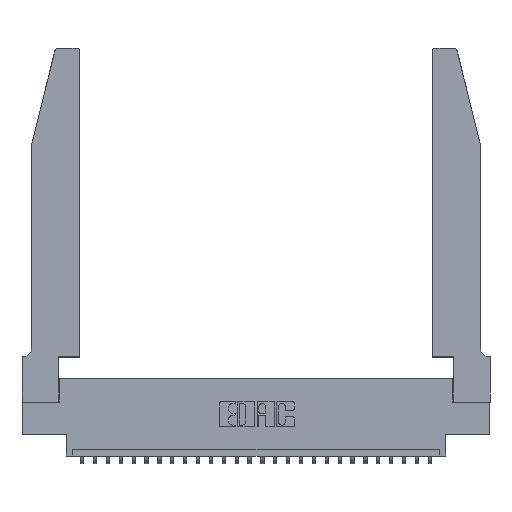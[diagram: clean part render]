
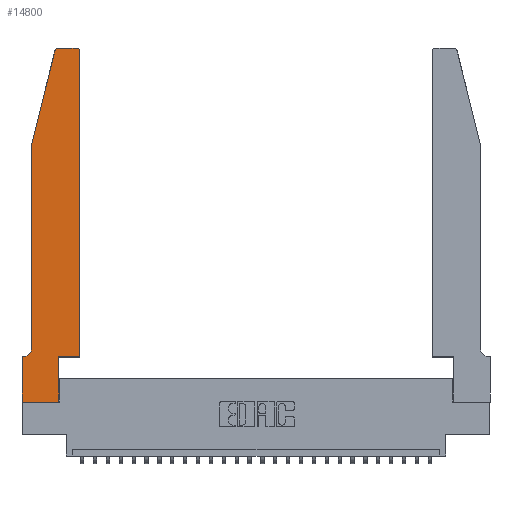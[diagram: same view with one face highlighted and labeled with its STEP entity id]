
A CAD part, top view. The second image highlights one B-rep face of the part: STEP entity #14800.
In plain terms, the highlighted planar face has unit normal (0, 0, 1).
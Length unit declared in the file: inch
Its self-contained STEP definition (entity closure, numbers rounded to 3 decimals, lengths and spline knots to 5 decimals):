
#120 = VERTEX_POINT ( 'NONE', #27929 ) ;
#493 = DIRECTION ( 'NONE',  ( 1., 0., 0. ) ) ;
#628 = ORIENTED_EDGE ( 'NONE', *, *, #4360, .T. ) ;
#676 = VERTEX_POINT ( 'NONE', #6365 ) ;
#863 = VECTOR ( 'NONE', #23464, 39.37008 ) ;
#1229 = DIRECTION ( 'NONE',  ( 0., 0., 1. ) ) ;
#1308 = LINE ( 'NONE', #25638, #17843 ) ;
#1491 = ORIENTED_EDGE ( 'NONE', *, *, #12616, .T. ) ;
#1509 = DIRECTION ( 'NONE',  ( 1., 0., 0. ) ) ;
#2576 = CARTESIAN_POINT ( 'NONE',  ( 0.0755, 2., 0.37 ) ) ;
#2586 = VECTOR ( 'NONE', #18319, 39.37008 ) ;
#2689 = ORIENTED_EDGE ( 'NONE', *, *, #12082, .T. ) ;
#2946 = EDGE_CURVE ( 'NONE', #13025, #27852, #9068, .T. ) ;
#3007 = VERTEX_POINT ( 'NONE', #10033 ) ;
#3605 = AXIS2_PLACEMENT_3D ( 'NONE', #23200, #27127, #16601 ) ;
#3829 = CARTESIAN_POINT ( 'NONE',  ( 0.4505, 0.35, 0.37 ) ) ;
#4138 = LINE ( 'NONE', #26491, #24666 ) ;
#4360 = EDGE_CURVE ( 'NONE', #27852, #14331, #20095, .T. ) ;
#4639 = EDGE_CURVE ( 'NONE', #3007, #13025, #23848, .T. ) ;
#4750 = ORIENTED_EDGE ( 'NONE', *, *, #19948, .T. ) ;
#5584 = VECTOR ( 'NONE', #7352, 39.37008 ) ;
#5677 = AXIS2_PLACEMENT_3D ( 'NONE', #24694, #15519, #15062 ) ;
#5797 = CARTESIAN_POINT ( 'NONE',  ( 0.4205, 2.75, 0.37 ) ) ;
#6245 = FACE_OUTER_BOUND ( 'NONE', #19116, .T. ) ;
#6365 = CARTESIAN_POINT ( 'NONE',  ( 0.2865, 0., 0.37 ) ) ;
#7292 = CARTESIAN_POINT ( 'NONE',  ( 0.0755, 2., 0.37 ) ) ;
#7317 = PLANE ( 'NONE',  #5677 ) ;
#7352 = DIRECTION ( 'NONE',  ( -1., 0., 0. ) ) ;
#7516 = CARTESIAN_POINT ( 'NONE',  ( 0.25487, 2.72718, 0.37 ) ) ;
#7613 = CARTESIAN_POINT ( 'NONE',  ( 0.284, 2.72, 0.37 ) ) ;
#7744 = CARTESIAN_POINT ( 'NONE',  ( 0.4505, 0.35, 0.37 ) ) ;
#7880 = ORIENTED_EDGE ( 'NONE', *, *, #16018, .T. ) ;
#7969 = VECTOR ( 'NONE', #20274, 39.37008 ) ;
#8444 = DIRECTION ( 'NONE',  ( 0., -1., 0. ) ) ;
#8537 = DIRECTION ( 'NONE',  ( 0., 1., 0. ) ) ;
#8971 = CIRCLE ( 'NONE', #3605, 0.07 ) ;
#9068 = LINE ( 'NONE', #3829, #20877 ) ;
#10033 = CARTESIAN_POINT ( 'NONE',  ( 0.2865, 0.35, 0.37 ) ) ;
#10373 = EDGE_CURVE ( 'NONE', #23273, #14984, #8971, .T. ) ;
#11060 = ORIENTED_EDGE ( 'NONE', *, *, #10373, .T. ) ;
#12082 = EDGE_CURVE ( 'NONE', #22036, #17152, #14065, .T. ) ;
#12116 = CARTESIAN_POINT ( 'NONE',  ( 0.2865, 0.35, 0.37 ) ) ;
#12616 = EDGE_CURVE ( 'NONE', #14984, #21402, #27543, .T. ) ;
#12976 = EDGE_CURVE ( 'NONE', #14331, #22036, #25532, .T. ) ;
#13025 = VERTEX_POINT ( 'NONE', #7744 ) ;
#14065 = CIRCLE ( 'NONE', #18116, 0.03 ) ;
#14331 = VERTEX_POINT ( 'NONE', #5797 ) ;
#14800 = ADVANCED_FACE ( 'NONE', ( #6245 ), #7317, .T. ) ;
#14984 = VERTEX_POINT ( 'NONE', #17025 ) ;
#15062 = DIRECTION ( 'NONE',  ( 1., 0., 0. ) ) ;
#15519 = DIRECTION ( 'NONE',  ( 0., 0., 1. ) ) ;
#15776 = CARTESIAN_POINT ( 'NONE',  ( 0.2605, 2.75, 0.37 ) ) ;
#16018 = EDGE_CURVE ( 'NONE', #120, #676, #4138, .T. ) ;
#16163 = ORIENTED_EDGE ( 'NONE', *, *, #12976, .T. ) ;
#16288 = VECTOR ( 'NONE', #8537, 39.37008 ) ;
#16416 = CARTESIAN_POINT ( 'NONE',  ( 0.4505, 2.72, 0.37 ) ) ;
#16601 = DIRECTION ( 'NONE',  ( -1., 0., 0. ) ) ;
#17025 = CARTESIAN_POINT ( 'NONE',  ( 0.0055, 0.35, 0.37 ) ) ;
#17152 = VERTEX_POINT ( 'NONE', #7516 ) ;
#17843 = VECTOR ( 'NONE', #8444, 39.37008 ) ;
#18116 = AXIS2_PLACEMENT_3D ( 'NONE', #7613, #1229, #22719 ) ;
#18319 = DIRECTION ( 'NONE',  ( 1., 0., 0. ) ) ;
#18626 = DIRECTION ( 'NONE',  ( 0., 1., 0. ) ) ;
#18630 = EDGE_CURVE ( 'NONE', #25165, #23273, #1308, .T. ) ;
#18834 = EDGE_CURVE ( 'NONE', #21402, #120, #25903, .T. ) ;
#18938 = CARTESIAN_POINT ( 'NONE',  ( 0., 0.35, 0.37 ) ) ;
#19116 = EDGE_LOOP ( 'NONE', ( #16163, #2689, #4750, #20839, #11060, #1491, #22860, #7880, #23858, #25107, #27418, #628 ) ) ;
#19539 = CARTESIAN_POINT ( 'NONE',  ( 0.0755, 0.42, 0.37 ) ) ;
#19948 = EDGE_CURVE ( 'NONE', #17152, #25165, #24495, .T. ) ;
#20079 = CARTESIAN_POINT ( 'NONE',  ( 0.4505, 0.35, 0.37 ) ) ;
#20095 = CIRCLE ( 'NONE', #26937, 0.03 ) ;
#20274 = DIRECTION ( 'NONE',  ( -1., 0., 0. ) ) ;
#20839 = ORIENTED_EDGE ( 'NONE', *, *, #18630, .T. ) ;
#20877 = VECTOR ( 'NONE', #18626, 39.37008 ) ;
#21402 = VERTEX_POINT ( 'NONE', #18938 ) ;
#22036 = VERTEX_POINT ( 'NONE', #26321 ) ;
#22173 = VECTOR ( 'NONE', #25368, 39.37008 ) ;
#22512 = EDGE_CURVE ( 'NONE', #676, #3007, #24046, .T. ) ;
#22719 = DIRECTION ( 'NONE',  ( 1., 0., 0. ) ) ;
#22860 = ORIENTED_EDGE ( 'NONE', *, *, #18834, .T. ) ;
#23102 = CARTESIAN_POINT ( 'NONE',  ( 0.4205, 2.72, 0.37 ) ) ;
#23200 = CARTESIAN_POINT ( 'NONE',  ( 0.0055, 0.42, 0.37 ) ) ;
#23221 = CARTESIAN_POINT ( 'NONE',  ( 0.0755, 0.35, 0.37 ) ) ;
#23273 = VERTEX_POINT ( 'NONE', #19539 ) ;
#23464 = DIRECTION ( 'NONE',  ( -0.239, -0.971, 0. ) ) ;
#23848 = LINE ( 'NONE', #20079, #2586 ) ;
#23858 = ORIENTED_EDGE ( 'NONE', *, *, #22512, .T. ) ;
#24046 = LINE ( 'NONE', #12116, #16288 ) ;
#24495 = LINE ( 'NONE', #2576, #863 ) ;
#24666 = VECTOR ( 'NONE', #493, 39.37008 ) ;
#24694 = CARTESIAN_POINT ( 'NONE',  ( 0., 0.35, 0.37 ) ) ;
#24869 = DIRECTION ( 'NONE',  ( 0., 0., 1. ) ) ;
#25107 = ORIENTED_EDGE ( 'NONE', *, *, #4639, .T. ) ;
#25165 = VERTEX_POINT ( 'NONE', #7292 ) ;
#25368 = DIRECTION ( 'NONE',  ( 0., -1., 0. ) ) ;
#25532 = LINE ( 'NONE', #15776, #5584 ) ;
#25638 = CARTESIAN_POINT ( 'NONE',  ( 0.0755, 2., 0.37 ) ) ;
#25903 = LINE ( 'NONE', #27903, #22173 ) ;
#26321 = CARTESIAN_POINT ( 'NONE',  ( 0.284, 2.75, 0.37 ) ) ;
#26491 = CARTESIAN_POINT ( 'NONE',  ( 0., 0., 0.37 ) ) ;
#26937 = AXIS2_PLACEMENT_3D ( 'NONE', #23102, #24869, #1509 ) ;
#27127 = DIRECTION ( 'NONE',  ( 0., 0., -1. ) ) ;
#27418 = ORIENTED_EDGE ( 'NONE', *, *, #2946, .T. ) ;
#27543 = LINE ( 'NONE', #23221, #7969 ) ;
#27852 = VERTEX_POINT ( 'NONE', #16416 ) ;
#27903 = CARTESIAN_POINT ( 'NONE',  ( 0., 0., 0.37 ) ) ;
#27929 = CARTESIAN_POINT ( 'NONE',  ( 0., 0., 0.37 ) ) ;
